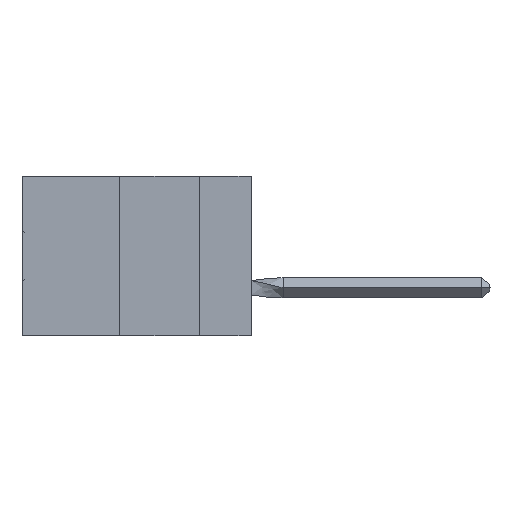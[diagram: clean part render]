
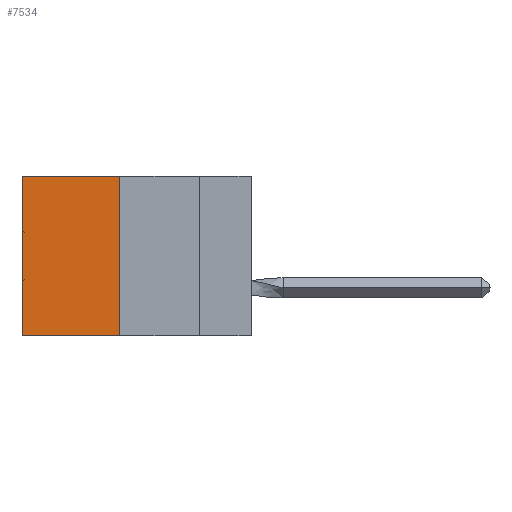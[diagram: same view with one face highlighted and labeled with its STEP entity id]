
A CAD part, left-side view. The second image highlights one B-rep face of the part: STEP entity #7534.
In plain terms, the highlighted planar face has unit normal (-1, 0, 0).
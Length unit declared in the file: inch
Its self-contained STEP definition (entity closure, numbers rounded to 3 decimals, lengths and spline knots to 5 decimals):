
#1890 = CARTESIAN_POINT ( 'NONE',  ( 0.305, 0.413, -0.5 ) ) ;
#3633 = DIRECTION ( 'NONE',  ( 1., 0., 0. ) ) ;
#4013 = DIRECTION ( 'NONE',  ( 0., 0., -1. ) ) ;
#4954 = VECTOR ( 'NONE', #50630, 39.37008 ) ;
#5222 = CARTESIAN_POINT ( 'NONE',  ( 0.305, 0.413, 0. ) ) ;
#6230 = VERTEX_POINT ( 'NONE', #25319 ) ;
#7534 = ADVANCED_FACE ( 'NONE', ( #38916 ), #28024, .F. ) ;
#7604 = CARTESIAN_POINT ( 'NONE',  ( 0.305, 0.413, -0.5 ) ) ;
#9674 = ORIENTED_EDGE ( 'NONE', *, *, #34898, .F. ) ;
#12673 = AXIS2_PLACEMENT_3D ( 'NONE', #7604, #3633, #4013 ) ;
#18211 = CARTESIAN_POINT ( 'NONE',  ( 0.305, 0.72, -0.5 ) ) ;
#22511 = DIRECTION ( 'NONE',  ( 0., 0., -1. ) ) ;
#22673 = CARTESIAN_POINT ( 'NONE',  ( 0.305, 0.72, -0.5 ) ) ;
#24356 = CARTESIAN_POINT ( 'NONE',  ( 0.305, 0.413, 0. ) ) ;
#24392 = EDGE_CURVE ( 'NONE', #28905, #30193, #48519, .T. ) ;
#25319 = CARTESIAN_POINT ( 'NONE',  ( 0.305, 0.413, -0.5 ) ) ;
#26279 = VERTEX_POINT ( 'NONE', #22673 ) ;
#28024 = PLANE ( 'NONE',  #12673 ) ;
#28905 = VERTEX_POINT ( 'NONE', #24356 ) ;
#29209 = LINE ( 'NONE', #1890, #37568 ) ;
#30193 = VERTEX_POINT ( 'NONE', #37562 ) ;
#33073 = EDGE_CURVE ( 'NONE', #30193, #26279, #49767, .T. ) ;
#34651 = DIRECTION ( 'NONE',  ( 0., 1., 0. ) ) ;
#34898 = EDGE_CURVE ( 'NONE', #28905, #6230, #36498, .T. ) ;
#36498 = LINE ( 'NONE', #36847, #50031 ) ;
#36847 = CARTESIAN_POINT ( 'NONE',  ( 0.305, 0.413, -0.5 ) ) ;
#37562 = CARTESIAN_POINT ( 'NONE',  ( 0.305, 0.72, 0. ) ) ;
#37568 = VECTOR ( 'NONE', #34651, 39.37008 ) ;
#38169 = VECTOR ( 'NONE', #22511, 39.37008 ) ;
#38916 = FACE_OUTER_BOUND ( 'NONE', #52400, .T. ) ;
#39179 = ORIENTED_EDGE ( 'NONE', *, *, #40579, .F. ) ;
#40579 = EDGE_CURVE ( 'NONE', #6230, #26279, #29209, .T. ) ;
#45362 = ORIENTED_EDGE ( 'NONE', *, *, #24392, .T. ) ;
#47856 = DIRECTION ( 'NONE',  ( 0., 0., -1. ) ) ;
#48519 = LINE ( 'NONE', #5222, #4954 ) ;
#48873 = ORIENTED_EDGE ( 'NONE', *, *, #33073, .T. ) ;
#49767 = LINE ( 'NONE', #18211, #38169 ) ;
#50031 = VECTOR ( 'NONE', #47856, 39.37008 ) ;
#50630 = DIRECTION ( 'NONE',  ( 0., 1., 0. ) ) ;
#52400 = EDGE_LOOP ( 'NONE', ( #48873, #39179, #9674, #45362 ) ) ;
